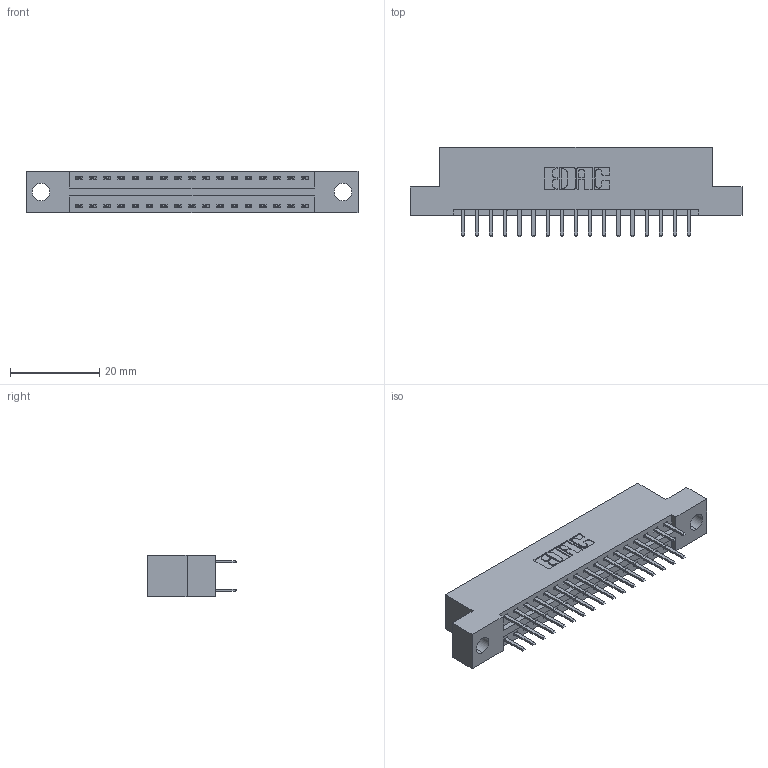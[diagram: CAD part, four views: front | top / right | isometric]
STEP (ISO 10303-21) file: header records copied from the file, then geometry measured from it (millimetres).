
FILE_DESCRIPTION (( 'STEP AP203' ), '1' );
FILE_NAME ('346-034-520-204.STEP', '2022-05-19T19:07:22', ( '' ), ( '' ), 'SwSTEP 2.0', 'SolidWorks 2020', '' );
FILE_SCHEMA (( 'CONFIG_CONTROL_DESIGN' ));
Length unit declared in the file: inch
Products named in the file (3): 345-292-001_345-293-120; 346-034-520-204; 346 Part_Flush Mounting Lugs - 0.156 Dia-TH
Assembly tree (35 placements, depth 2):
  346-034-520-204
    346 Part_Flush Mounting Lugs - 0.156 Dia-TH
    345-292-001_345-293-120  x34
Bounding box: 74.55 x 20.02 x 9.4 mm (x, y, z)
Volume: 6954.4 mm3; surface area: 8979.2 mm2
Topology: 35 solids, 35 shells, 2040 faces, 5907 edges, 3846 vertices
Faces by surface type: plane 1348, cylinder 692
Entity records: 14993 total; most frequent: CARTESIAN_POINT 2522, ORIENTED_EDGE 2442, DIRECTION 2261, EDGE_CURVE 1221, VECTOR 1017, LINE 1017, VERTEX_POINT 810, AXIS2_PLACEMENT_3D 622
